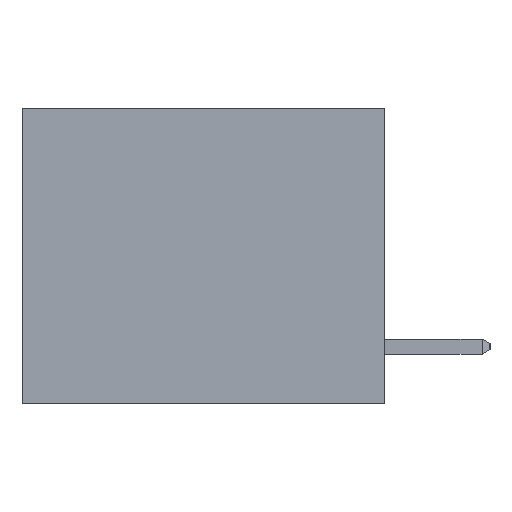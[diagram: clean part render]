
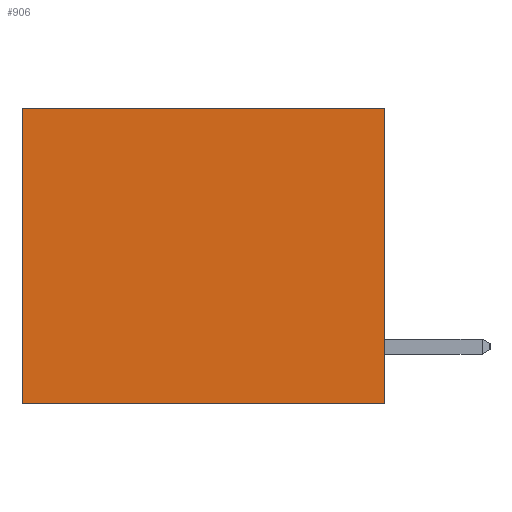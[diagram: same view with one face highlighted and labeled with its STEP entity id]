
A CAD part, left-side view. The second image highlights one B-rep face of the part: STEP entity #906.
In plain terms, the highlighted planar face has unit normal (-1, 0, 0).
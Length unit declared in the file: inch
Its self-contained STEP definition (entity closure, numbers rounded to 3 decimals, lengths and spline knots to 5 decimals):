
#6 = CARTESIAN_POINT ( 'NONE',  ( 0.3165, 0., -0.49 ) ) ;
#689 = VERTEX_POINT ( 'NONE', #21253 ) ;
#906 = ADVANCED_FACE ( 'NONE', ( #1964 ), #10738, .F. ) ;
#1595 = LINE ( 'NONE', #10210, #14587 ) ;
#1964 = FACE_OUTER_BOUND ( 'NONE', #10010, .T. ) ;
#2632 = EDGE_CURVE ( 'NONE', #689, #8822, #19824, .T. ) ;
#2830 = VECTOR ( 'NONE', #18281, 39.37008 ) ;
#3605 = CARTESIAN_POINT ( 'NONE',  ( 0.3165, 0.6, 0. ) ) ;
#3717 = ORIENTED_EDGE ( 'NONE', *, *, #2632, .T. ) ;
#4684 = EDGE_CURVE ( 'NONE', #689, #10003, #6773, .T. ) ;
#5020 = ORIENTED_EDGE ( 'NONE', *, *, #4684, .F. ) ;
#6039 = CARTESIAN_POINT ( 'NONE',  ( 0.3165, 0., 0. ) ) ;
#6773 = LINE ( 'NONE', #21364, #2830 ) ;
#7821 = CARTESIAN_POINT ( 'NONE',  ( 0.3165, 0., -0.49 ) ) ;
#8035 = DIRECTION ( 'NONE',  ( 0., 1., 0. ) ) ;
#8546 = DIRECTION ( 'NONE',  ( 1., 0., 0. ) ) ;
#8822 = VERTEX_POINT ( 'NONE', #3605 ) ;
#9071 = VECTOR ( 'NONE', #9735, 39.37008 ) ;
#9624 = AXIS2_PLACEMENT_3D ( 'NONE', #12668, #8546, #14443 ) ;
#9735 = DIRECTION ( 'NONE',  ( 0., 1., 0. ) ) ;
#10003 = VERTEX_POINT ( 'NONE', #7821 ) ;
#10010 = EDGE_LOOP ( 'NONE', ( #11339, #22257, #5020, #3717 ) ) ;
#10210 = CARTESIAN_POINT ( 'NONE',  ( 0.3165, 0.6, -0.49 ) ) ;
#10738 = PLANE ( 'NONE',  #9624 ) ;
#11339 = ORIENTED_EDGE ( 'NONE', *, *, #17382, .T. ) ;
#11385 = VECTOR ( 'NONE', #8035, 39.37008 ) ;
#12668 = CARTESIAN_POINT ( 'NONE',  ( 0.3165, 0., -0.49 ) ) ;
#13313 = LINE ( 'NONE', #6, #9071 ) ;
#14443 = DIRECTION ( 'NONE',  ( 0., 0., -1. ) ) ;
#14587 = VECTOR ( 'NONE', #20060, 39.37008 ) ;
#17382 = EDGE_CURVE ( 'NONE', #8822, #22908, #1595, .T. ) ;
#18281 = DIRECTION ( 'NONE',  ( 0., 0., -1. ) ) ;
#19824 = LINE ( 'NONE', #6039, #11385 ) ;
#20060 = DIRECTION ( 'NONE',  ( 0., 0., -1. ) ) ;
#21003 = CARTESIAN_POINT ( 'NONE',  ( 0.3165, 0.6, -0.49 ) ) ;
#21253 = CARTESIAN_POINT ( 'NONE',  ( 0.3165, 0., 0. ) ) ;
#21364 = CARTESIAN_POINT ( 'NONE',  ( 0.3165, 0., -0.49 ) ) ;
#22257 = ORIENTED_EDGE ( 'NONE', *, *, #22991, .F. ) ;
#22908 = VERTEX_POINT ( 'NONE', #21003 ) ;
#22991 = EDGE_CURVE ( 'NONE', #10003, #22908, #13313, .T. ) ;
